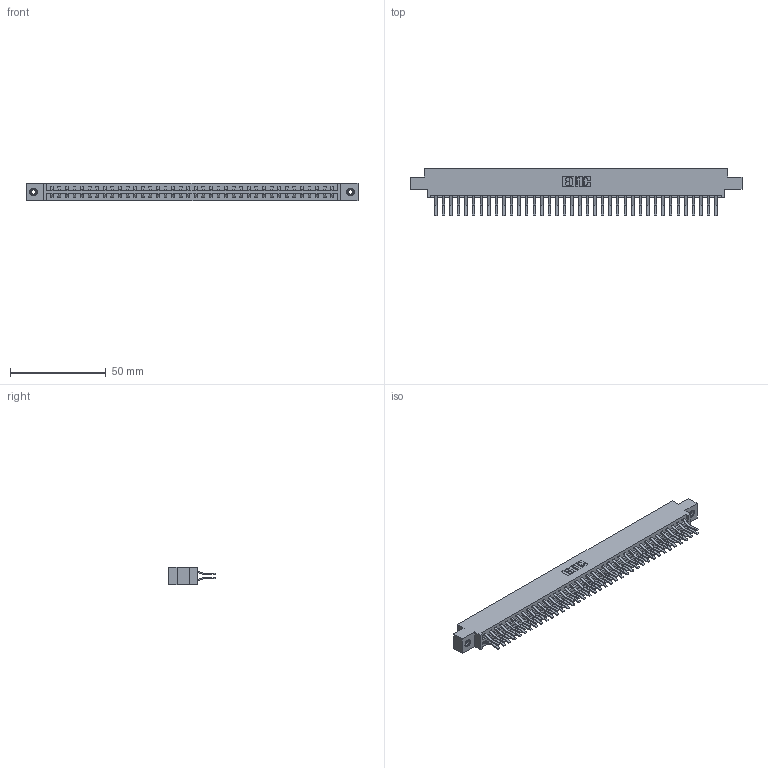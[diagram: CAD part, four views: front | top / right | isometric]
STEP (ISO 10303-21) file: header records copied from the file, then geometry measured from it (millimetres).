
FILE_DESCRIPTION (( 'STEP AP203' ), '1' );
FILE_NAME ('337-076-560-808.STEP', '2018-08-12T15:09:00', ( '' ), ( '' ), 'SwSTEP 2.0', 'SolidWorks 2016', '' );
FILE_SCHEMA (( 'CONFIG_CONTROL_DESIGN' ));
Length unit declared in the file: inch
Products named in the file (4): 337 Part_0.170 Offset - 0.156 Dia-TI; 345-292-001_560 Tail; 345-250-001_345-250-003-102; 337-076-560-808
Assembly tree (79 placements, depth 2):
  337-076-560-808
    337 Part_0.170 Offset - 0.156 Dia-TI
    345-292-001_560 Tail  x76
    345-250-001_345-250-003-102  x2
Bounding box: 173.58 x 24.78 x 9.4 mm (x, y, z)
Volume: 18614.5 mm3; surface area: 22578.4 mm2
Topology: 79 solids, 79 shells, 4434 faces, 13151 edges, 8658 vertices
Faces by surface type: plane 2994, cylinder 1424, cone 12, torus 4
Entity records: 31386 total; most frequent: CARTESIAN_POINT 5273, ORIENTED_EDGE 5202, DIRECTION 4527, EDGE_CURVE 2601, VECTOR 2449, LINE 2449, VERTEX_POINT 1728, AXIS2_PLACEMENT_3D 1039
